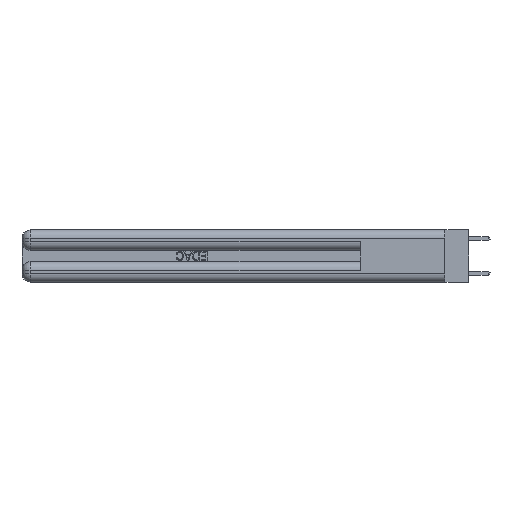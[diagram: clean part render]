
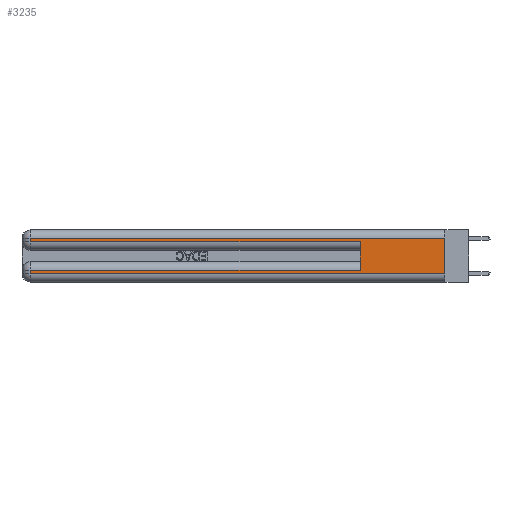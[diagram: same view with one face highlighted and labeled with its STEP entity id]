
A CAD part, left-side view. The second image highlights one B-rep face of the part: STEP entity #3235.
In plain terms, the highlighted planar face has unit normal (-1, 0, 0).
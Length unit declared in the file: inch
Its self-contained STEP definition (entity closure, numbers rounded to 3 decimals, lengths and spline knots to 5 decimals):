
#246 = CARTESIAN_POINT ( 'NONE',  ( 0., 2.94, 0.06 ) ) ;
#332 = VECTOR ( 'NONE', #10327, 39.37008 ) ;
#611 = ORIENTED_EDGE ( 'NONE', *, *, #21604, .T. ) ;
#1272 = FACE_OUTER_BOUND ( 'NONE', #5019, .T. ) ;
#1465 = LINE ( 'NONE', #8911, #11777 ) ;
#1876 = LINE ( 'NONE', #4626, #9319 ) ;
#2228 = DIRECTION ( 'NONE',  ( 0., 0., -1. ) ) ;
#2680 = EDGE_CURVE ( 'NONE', #3470, #6771, #31060, .T. ) ;
#2943 = EDGE_CURVE ( 'NONE', #6771, #27886, #5109, .T. ) ;
#3235 = ADVANCED_FACE ( 'NONE', ( #1272 ), #4541, .F. ) ;
#3470 = VERTEX_POINT ( 'NONE', #16963 ) ;
#3647 = EDGE_CURVE ( 'NONE', #23395, #21972, #1876, .T. ) ;
#3649 = DIRECTION ( 'NONE',  ( 0., -1., 0. ) ) ;
#4526 = CARTESIAN_POINT ( 'NONE',  ( 0., 0., 0.085 ) ) ;
#4541 = PLANE ( 'NONE',  #32429 ) ;
#4626 = CARTESIAN_POINT ( 'NONE',  ( 0., 0., 0.37 ) ) ;
#4849 = ORIENTED_EDGE ( 'NONE', *, *, #20158, .T. ) ;
#5019 = EDGE_LOOP ( 'NONE', ( #10458, #4849, #17626, #611, #10569, #12002, #7373, #26851 ) ) ;
#5109 = LINE ( 'NONE', #31469, #332 ) ;
#5301 = VECTOR ( 'NONE', #28273, 39.37008 ) ;
#6771 = VERTEX_POINT ( 'NONE', #9335 ) ;
#7373 = ORIENTED_EDGE ( 'NONE', *, *, #2943, .T. ) ;
#7587 = VERTEX_POINT ( 'NONE', #8671 ) ;
#8610 = DIRECTION ( 'NONE',  ( 0., 0., 1. ) ) ;
#8671 = CARTESIAN_POINT ( 'NONE',  ( 0., 0.6, 0.285 ) ) ;
#8911 = CARTESIAN_POINT ( 'NONE',  ( 0., 2.94, 0.37 ) ) ;
#9319 = VECTOR ( 'NONE', #2228, 39.37008 ) ;
#9335 = CARTESIAN_POINT ( 'NONE',  ( 0., 2.94, 0.085 ) ) ;
#9717 = CARTESIAN_POINT ( 'NONE',  ( 0., 0., 0.06 ) ) ;
#9752 = CARTESIAN_POINT ( 'NONE',  ( 0., 0., 0.37 ) ) ;
#10327 = DIRECTION ( 'NONE',  ( 0., 0., -1. ) ) ;
#10458 = ORIENTED_EDGE ( 'NONE', *, *, #3647, .F. ) ;
#10569 = ORIENTED_EDGE ( 'NONE', *, *, #25181, .F. ) ;
#11777 = VECTOR ( 'NONE', #17060, 39.37008 ) ;
#12002 = ORIENTED_EDGE ( 'NONE', *, *, #2680, .T. ) ;
#13913 = LINE ( 'NONE', #30199, #20721 ) ;
#13982 = CARTESIAN_POINT ( 'NONE',  ( 0., 0.6, 0.145 ) ) ;
#16963 = CARTESIAN_POINT ( 'NONE',  ( 0., 0.6, 0.085 ) ) ;
#17060 = DIRECTION ( 'NONE',  ( 0., 0., -1. ) ) ;
#17560 = VERTEX_POINT ( 'NONE', #27440 ) ;
#17626 = ORIENTED_EDGE ( 'NONE', *, *, #18883, .T. ) ;
#18883 = EDGE_CURVE ( 'NONE', #21518, #17560, #1465, .T. ) ;
#19988 = DIRECTION ( 'NONE',  ( 0., 0., -1. ) ) ;
#20158 = EDGE_CURVE ( 'NONE', #23395, #21518, #13913, .T. ) ;
#20721 = VECTOR ( 'NONE', #24467, 39.37008 ) ;
#21518 = VERTEX_POINT ( 'NONE', #25027 ) ;
#21604 = EDGE_CURVE ( 'NONE', #17560, #7587, #23078, .T. ) ;
#21972 = VERTEX_POINT ( 'NONE', #22190 ) ;
#22190 = CARTESIAN_POINT ( 'NONE',  ( 0., 0., 0.06 ) ) ;
#23078 = LINE ( 'NONE', #33657, #25063 ) ;
#23091 = DIRECTION ( 'NONE',  ( 1., 0., 0. ) ) ;
#23254 = DIRECTION ( 'NONE',  ( 0., -1., 0. ) ) ;
#23395 = VERTEX_POINT ( 'NONE', #33325 ) ;
#24467 = DIRECTION ( 'NONE',  ( 0., 1., 0. ) ) ;
#24961 = VECTOR ( 'NONE', #8610, 39.37008 ) ;
#25027 = CARTESIAN_POINT ( 'NONE',  ( 0., 2.94, 0.31 ) ) ;
#25063 = VECTOR ( 'NONE', #23254, 39.37008 ) ;
#25181 = EDGE_CURVE ( 'NONE', #3470, #7587, #32358, .T. ) ;
#26851 = ORIENTED_EDGE ( 'NONE', *, *, #33919, .T. ) ;
#27440 = CARTESIAN_POINT ( 'NONE',  ( 0., 2.94, 0.285 ) ) ;
#27886 = VERTEX_POINT ( 'NONE', #246 ) ;
#28273 = DIRECTION ( 'NONE',  ( 0., 1., 0. ) ) ;
#30193 = VECTOR ( 'NONE', #3649, 39.37008 ) ;
#30199 = CARTESIAN_POINT ( 'NONE',  ( 0., 0., 0.31 ) ) ;
#31060 = LINE ( 'NONE', #4526, #5301 ) ;
#31469 = CARTESIAN_POINT ( 'NONE',  ( 0., 2.94, 0.37 ) ) ;
#32358 = LINE ( 'NONE', #13982, #24961 ) ;
#32429 = AXIS2_PLACEMENT_3D ( 'NONE', #9752, #23091, #19988 ) ;
#32947 = LINE ( 'NONE', #9717, #30193 ) ;
#33325 = CARTESIAN_POINT ( 'NONE',  ( 0., 0., 0.31 ) ) ;
#33657 = CARTESIAN_POINT ( 'NONE',  ( 0., 0., 0.285 ) ) ;
#33919 = EDGE_CURVE ( 'NONE', #27886, #21972, #32947, .T. ) ;
